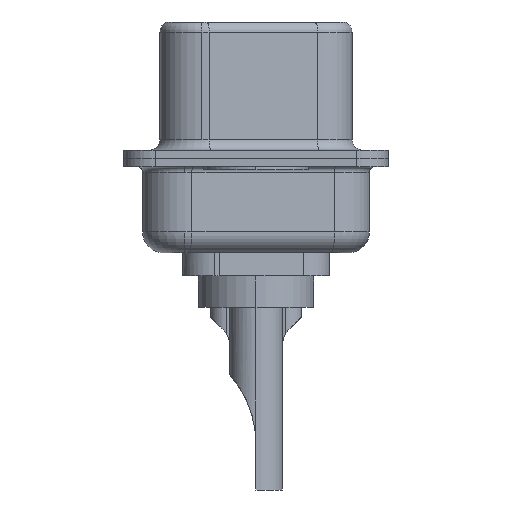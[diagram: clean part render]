
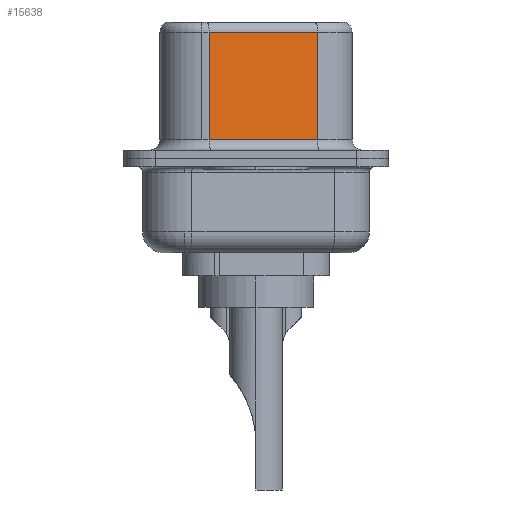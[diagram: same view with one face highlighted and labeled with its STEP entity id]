
A CAD part, left-side view. The second image highlights one B-rep face of the part: STEP entity #15638.
In plain terms, the highlighted planar face has unit normal (-0.985, -0.174, 0).
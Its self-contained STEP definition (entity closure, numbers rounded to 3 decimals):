
#45 = CARTESIAN_POINT ( 'NONE',  ( 4.585, -2.927, 6.52 ) ) ;
#146 = LINE ( 'NONE', #8213, #5574 ) ;
#218 = CARTESIAN_POINT ( 'NONE',  ( 3.675, 2.233, 6.02 ) ) ;
#1403 = LINE ( 'NONE', #4826, #11982 ) ;
#2292 = ORIENTED_EDGE ( 'NONE', *, *, #4287, .T. ) ;
#2931 = VERTEX_POINT ( 'NONE', #5453 ) ;
#3224 = VECTOR ( 'NONE', #10096, 1000. ) ;
#3385 = VECTOR ( 'NONE', #5330, 1000. ) ;
#4052 = EDGE_CURVE ( 'NONE', #17156, #2931, #146, .T. ) ;
#4128 = FACE_OUTER_BOUND ( 'NONE', #14388, .T. ) ;
#4287 = EDGE_CURVE ( 'NONE', #8548, #2931, #9852, .T. ) ;
#4298 = DIRECTION ( 'NONE',  ( -0.174, 0.985, 0. ) ) ;
#4576 = EDGE_CURVE ( 'NONE', #10834, #8548, #1403, .T. ) ;
#4826 = CARTESIAN_POINT ( 'NONE',  ( 3.675, 2.233, 6.52 ) ) ;
#5330 = DIRECTION ( 'NONE',  ( 0.174, -0.985, 0. ) ) ;
#5453 = CARTESIAN_POINT ( 'NONE',  ( 4.585, -2.927, 0.9 ) ) ;
#5486 = EDGE_CURVE ( 'NONE', #17156, #10834, #13322, .T. ) ;
#5574 = VECTOR ( 'NONE', #16244, 1000. ) ;
#6649 = CARTESIAN_POINT ( 'NONE',  ( 4.585, -2.927, 0.9 ) ) ;
#7060 = PLANE ( 'NONE',  #17859 ) ;
#7263 = CARTESIAN_POINT ( 'NONE',  ( 4.585, -2.927, 6.02 ) ) ;
#8213 = CARTESIAN_POINT ( 'NONE',  ( 4.585, -2.927, 6.52 ) ) ;
#8548 = VERTEX_POINT ( 'NONE', #16663 ) ;
#9415 = CARTESIAN_POINT ( 'NONE',  ( 4.585, -2.927, 6.02 ) ) ;
#9852 = LINE ( 'NONE', #6649, #3385 ) ;
#10096 = DIRECTION ( 'NONE',  ( -0.174, 0.985, 0. ) ) ;
#10834 = VERTEX_POINT ( 'NONE', #218 ) ;
#10953 = ORIENTED_EDGE ( 'NONE', *, *, #5486, .T. ) ;
#11982 = VECTOR ( 'NONE', #14441, 1000. ) ;
#13322 = LINE ( 'NONE', #7263, #3224 ) ;
#14168 = ORIENTED_EDGE ( 'NONE', *, *, #4576, .T. ) ;
#14388 = EDGE_LOOP ( 'NONE', ( #15812, #10953, #14168, #2292 ) ) ;
#14441 = DIRECTION ( 'NONE',  ( 0., 0., -1. ) ) ;
#15638 = ADVANCED_FACE ( 'NONE', ( #4128 ), #7060, .F. ) ;
#15812 = ORIENTED_EDGE ( 'NONE', *, *, #4052, .F. ) ;
#16244 = DIRECTION ( 'NONE',  ( 0., 0., -1. ) ) ;
#16556 = DIRECTION ( 'NONE',  ( 0.985, 0.174, 0. ) ) ;
#16663 = CARTESIAN_POINT ( 'NONE',  ( 3.675, 2.233, 0.9 ) ) ;
#17156 = VERTEX_POINT ( 'NONE', #9415 ) ;
#17859 = AXIS2_PLACEMENT_3D ( 'NONE', #45, #16556, #4298 ) ;
